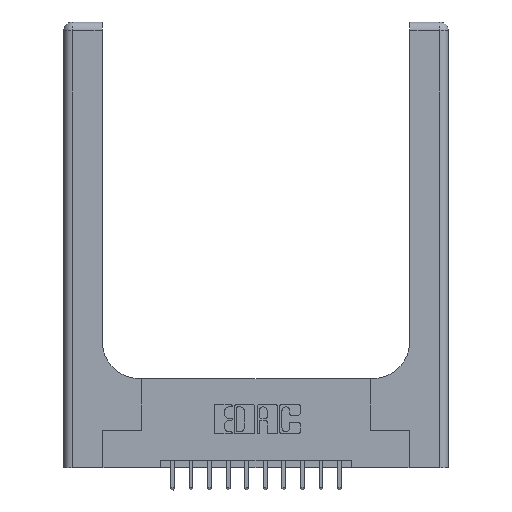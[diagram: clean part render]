
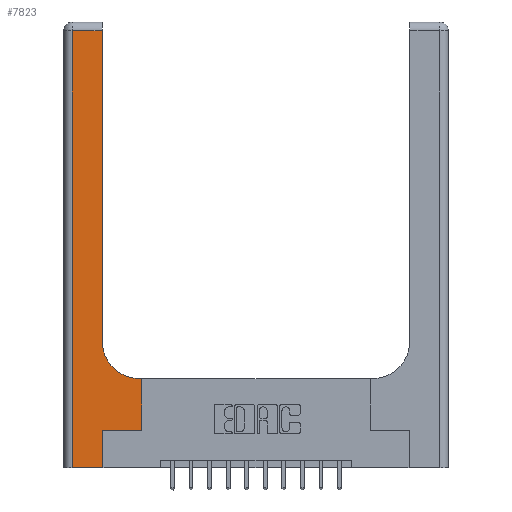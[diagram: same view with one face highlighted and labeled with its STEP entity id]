
A CAD part, top view. The second image highlights one B-rep face of the part: STEP entity #7823.
In plain terms, the highlighted planar face has unit normal (0, 0, 1).
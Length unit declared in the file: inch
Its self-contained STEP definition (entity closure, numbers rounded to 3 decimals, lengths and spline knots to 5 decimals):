
#65 = VECTOR ( 'NONE', #4735, 39.37008 ) ;
#70 = VERTEX_POINT ( 'NONE', #3003 ) ;
#137 = VECTOR ( 'NONE', #1124, 39.37008 ) ;
#536 = VERTEX_POINT ( 'NONE', #8970 ) ;
#860 = LINE ( 'NONE', #6372, #2770 ) ;
#984 = EDGE_CURVE ( 'NONE', #8506, #70, #11404, .T. ) ;
#1124 = DIRECTION ( 'NONE',  ( 1., 0., 0. ) ) ;
#1155 = DIRECTION ( 'NONE',  ( 0., 1., 0. ) ) ;
#1195 = VERTEX_POINT ( 'NONE', #8982 ) ;
#1215 = VERTEX_POINT ( 'NONE', #2877 ) ;
#1439 = CARTESIAN_POINT ( 'NONE',  ( 0.26, 0.85, 0.37 ) ) ;
#1479 = DIRECTION ( 'NONE',  ( 0., 0., -1. ) ) ;
#1649 = CARTESIAN_POINT ( 'NONE',  ( 0.26, 2.94, 0.37 ) ) ;
#1798 = ORIENTED_EDGE ( 'NONE', *, *, #984, .T. ) ;
#1914 = VECTOR ( 'NONE', #6448, 39.37008 ) ;
#2163 = LINE ( 'NONE', #2930, #3109 ) ;
#2356 = VECTOR ( 'NONE', #1155, 39.37008 ) ;
#2389 = LINE ( 'NONE', #12286, #65 ) ;
#2556 = CARTESIAN_POINT ( 'NONE',  ( 0.265, 0.25, 0.37 ) ) ;
#2759 = PLANE ( 'NONE',  #12108 ) ;
#2770 = VECTOR ( 'NONE', #8742, 39.37008 ) ;
#2877 = CARTESIAN_POINT ( 'NONE',  ( 0.51, 0.6, 0.37 ) ) ;
#2930 = CARTESIAN_POINT ( 'NONE',  ( 0.26, 0.6, 0.37 ) ) ;
#2959 = ORIENTED_EDGE ( 'NONE', *, *, #11449, .T. ) ;
#3003 = CARTESIAN_POINT ( 'NONE',  ( 0.528, 0.25, 0.37 ) ) ;
#3109 = VECTOR ( 'NONE', #15116, 39.37008 ) ;
#3123 = LINE ( 'NONE', #12359, #12291 ) ;
#3637 = LINE ( 'NONE', #15701, #13960 ) ;
#4069 = EDGE_CURVE ( 'NONE', #536, #1215, #2163, .T. ) ;
#4735 = DIRECTION ( 'NONE',  ( -1., 0., 0. ) ) ;
#5045 = CARTESIAN_POINT ( 'NONE',  ( 0.06, 2.94, 0.37 ) ) ;
#6372 = CARTESIAN_POINT ( 'NONE',  ( 0.265, 0., 0.37 ) ) ;
#6429 = DIRECTION ( 'NONE',  ( -1., 0., 0. ) ) ;
#6448 = DIRECTION ( 'NONE',  ( 1., 0., 0. ) ) ;
#6464 = LINE ( 'NONE', #8596, #2356 ) ;
#6584 = VERTEX_POINT ( 'NONE', #7372 ) ;
#6661 = DIRECTION ( 'NONE',  ( 1., 0., 0. ) ) ;
#7172 = DIRECTION ( 'NONE',  ( 0., -1., 0. ) ) ;
#7260 = EDGE_CURVE ( 'NONE', #1195, #6584, #7729, .T. ) ;
#7268 = DIRECTION ( 'NONE',  ( 0., 1., 0. ) ) ;
#7372 = CARTESIAN_POINT ( 'NONE',  ( 0.265, 0., 0.37 ) ) ;
#7729 = LINE ( 'NONE', #11440, #1914 ) ;
#7823 = ADVANCED_FACE ( 'NONE', ( #10047 ), #2759, .F. ) ;
#7881 = ORIENTED_EDGE ( 'NONE', *, *, #8606, .T. ) ;
#8007 = DIRECTION ( 'NONE',  ( 0., 0., -1. ) ) ;
#8506 = VERTEX_POINT ( 'NONE', #2556 ) ;
#8596 = CARTESIAN_POINT ( 'NONE',  ( 0.528, 0.25, 0.37 ) ) ;
#8606 = EDGE_CURVE ( 'NONE', #1215, #9399, #10243, .T. ) ;
#8660 = ORIENTED_EDGE ( 'NONE', *, *, #11447, .T. ) ;
#8742 = DIRECTION ( 'NONE',  ( 0., 1., 0. ) ) ;
#8826 = CARTESIAN_POINT ( 'NONE',  ( 0.265, 0.25, 0.37 ) ) ;
#8970 = CARTESIAN_POINT ( 'NONE',  ( 0.528, 0.6, 0.37 ) ) ;
#8982 = CARTESIAN_POINT ( 'NONE',  ( 0.06, 0., 0.37 ) ) ;
#9108 = AXIS2_PLACEMENT_3D ( 'NONE', #14095, #8007, #6661 ) ;
#9399 = VERTEX_POINT ( 'NONE', #1439 ) ;
#9637 = ORIENTED_EDGE ( 'NONE', *, *, #10639, .T. ) ;
#10047 = FACE_OUTER_BOUND ( 'NONE', #14756, .T. ) ;
#10243 = CIRCLE ( 'NONE', #9108, 0.25 ) ;
#10639 = EDGE_CURVE ( 'NONE', #11814, #10818, #2389, .T. ) ;
#10810 = EDGE_CURVE ( 'NONE', #6584, #8506, #860, .T. ) ;
#10818 = VERTEX_POINT ( 'NONE', #5045 ) ;
#11404 = LINE ( 'NONE', #8826, #137 ) ;
#11440 = CARTESIAN_POINT ( 'NONE',  ( 0., 0., 0.37 ) ) ;
#11447 = EDGE_CURVE ( 'NONE', #9399, #11814, #3123, .T. ) ;
#11449 = EDGE_CURVE ( 'NONE', #70, #536, #6464, .T. ) ;
#11814 = VERTEX_POINT ( 'NONE', #1649 ) ;
#12108 = AXIS2_PLACEMENT_3D ( 'NONE', #12711, #1479, #6429 ) ;
#12286 = CARTESIAN_POINT ( 'NONE',  ( 0., 2.94, 0.37 ) ) ;
#12291 = VECTOR ( 'NONE', #7268, 39.37008 ) ;
#12359 = CARTESIAN_POINT ( 'NONE',  ( 0.26, 3., 0.37 ) ) ;
#12711 = CARTESIAN_POINT ( 'NONE',  ( 0., 3., 0.37 ) ) ;
#13133 = ORIENTED_EDGE ( 'NONE', *, *, #10810, .T. ) ;
#13255 = ORIENTED_EDGE ( 'NONE', *, *, #7260, .T. ) ;
#13830 = ORIENTED_EDGE ( 'NONE', *, *, #14032, .T. ) ;
#13960 = VECTOR ( 'NONE', #7172, 39.37008 ) ;
#14032 = EDGE_CURVE ( 'NONE', #10818, #1195, #3637, .T. ) ;
#14095 = CARTESIAN_POINT ( 'NONE',  ( 0.51, 0.85, 0.37 ) ) ;
#14756 = EDGE_LOOP ( 'NONE', ( #8660, #9637, #13830, #13255, #13133, #1798, #2959, #15639, #7881 ) ) ;
#15116 = DIRECTION ( 'NONE',  ( -1., 0., 0. ) ) ;
#15639 = ORIENTED_EDGE ( 'NONE', *, *, #4069, .T. ) ;
#15701 = CARTESIAN_POINT ( 'NONE',  ( 0.06, 3., 0.37 ) ) ;
